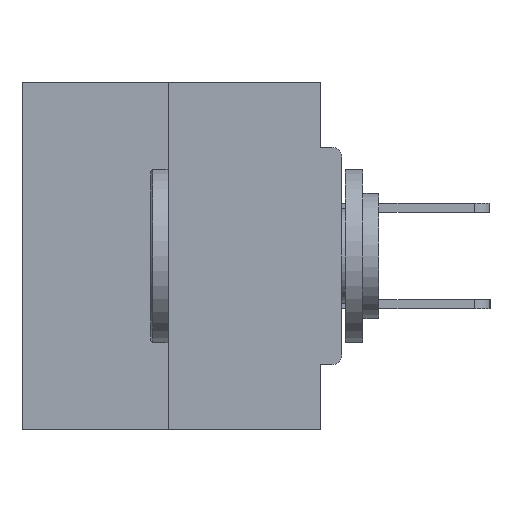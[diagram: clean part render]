
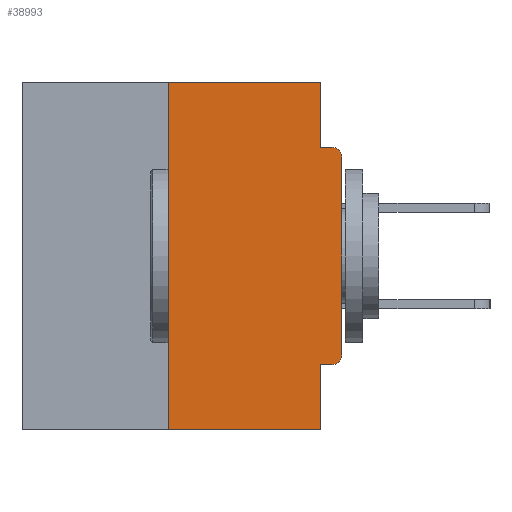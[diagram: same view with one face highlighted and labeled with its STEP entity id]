
A CAD part, left-side view. The second image highlights one B-rep face of the part: STEP entity #38993.
In plain terms, the highlighted planar face has unit normal (-1, 0, 0).
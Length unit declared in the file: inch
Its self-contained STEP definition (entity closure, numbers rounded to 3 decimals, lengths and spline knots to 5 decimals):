
#221 = ORIENTED_EDGE ( 'NONE', *, *, #35527, .T. ) ;
#1279 = ORIENTED_EDGE ( 'NONE', *, *, #10963, .F. ) ;
#2219 = CARTESIAN_POINT ( 'NONE',  ( 0., 0.46, 0. ) ) ;
#2392 = VERTEX_POINT ( 'NONE', #35817 ) ;
#2766 = EDGE_CURVE ( 'NONE', #2392, #14048, #25128, .T. ) ;
#2801 = CIRCLE ( 'NONE', #18973, 0.015 ) ;
#2905 = CARTESIAN_POINT ( 'NONE',  ( 0., 0., 0. ) ) ;
#4479 = ORIENTED_EDGE ( 'NONE', *, *, #8475, .F. ) ;
#4481 = CARTESIAN_POINT ( 'NONE',  ( 0., 0.015, -0.3915 ) ) ;
#5350 = ORIENTED_EDGE ( 'NONE', *, *, #27607, .T. ) ;
#5554 = FACE_OUTER_BOUND ( 'NONE', #33167, .T. ) ;
#7343 = CARTESIAN_POINT ( 'NONE',  ( 0., 0.015, -0.0935 ) ) ;
#8475 = EDGE_CURVE ( 'NONE', #9033, #37160, #33747, .T. ) ;
#9033 = VERTEX_POINT ( 'NONE', #37750 ) ;
#10115 = DIRECTION ( 'NONE',  ( 0., 0., -1. ) ) ;
#10771 = DIRECTION ( 'NONE',  ( 0., 1., 0. ) ) ;
#10941 = DIRECTION ( 'NONE',  ( 0., 0., -1. ) ) ;
#10963 = EDGE_CURVE ( 'NONE', #17591, #20690, #32043, .T. ) ;
#11376 = LINE ( 'NONE', #23255, #17923 ) ;
#11535 = EDGE_CURVE ( 'NONE', #39991, #20321, #31551, .T. ) ;
#11856 = CARTESIAN_POINT ( 'NONE',  ( 0., 0.031, -0.5 ) ) ;
#12567 = ORIENTED_EDGE ( 'NONE', *, *, #33203, .F. ) ;
#12616 = DIRECTION ( 'NONE',  ( 0., 0., -1. ) ) ;
#12732 = DIRECTION ( 'NONE',  ( 0., 0., -1. ) ) ;
#12883 = CARTESIAN_POINT ( 'NONE',  ( 0., 0.031, 0. ) ) ;
#13154 = AXIS2_PLACEMENT_3D ( 'NONE', #2219, #15579, #12732 ) ;
#13315 = DIRECTION ( 'NONE',  ( 0., 0., 1. ) ) ;
#13701 = CARTESIAN_POINT ( 'NONE',  ( 0., 0.015, -0.4065 ) ) ;
#13846 = EDGE_CURVE ( 'NONE', #20321, #39952, #15249, .T. ) ;
#14048 = VERTEX_POINT ( 'NONE', #7343 ) ;
#15249 = LINE ( 'NONE', #2905, #29307 ) ;
#15579 = DIRECTION ( 'NONE',  ( 1., 0., 0. ) ) ;
#15753 = CARTESIAN_POINT ( 'NONE',  ( 0., 0., -0.0935 ) ) ;
#15864 = CARTESIAN_POINT ( 'NONE',  ( 0., 0.25, -0.5 ) ) ;
#15927 = ORIENTED_EDGE ( 'NONE', *, *, #2766, .F. ) ;
#17042 = VECTOR ( 'NONE', #32175, 39.37008 ) ;
#17215 = VECTOR ( 'NONE', #10771, 39.37008 ) ;
#17591 = VERTEX_POINT ( 'NONE', #15864 ) ;
#17923 = VECTOR ( 'NONE', #10115, 39.37008 ) ;
#18106 = PLANE ( 'NONE',  #13154 ) ;
#18656 = CARTESIAN_POINT ( 'NONE',  ( 0., 0.015, -0.1085 ) ) ;
#18973 = AXIS2_PLACEMENT_3D ( 'NONE', #18656, #25163, #12616 ) ;
#19751 = LINE ( 'NONE', #40129, #17215 ) ;
#20080 = ORIENTED_EDGE ( 'NONE', *, *, #13846, .T. ) ;
#20321 = VERTEX_POINT ( 'NONE', #40772 ) ;
#20690 = VERTEX_POINT ( 'NONE', #23132 ) ;
#21570 = CARTESIAN_POINT ( 'NONE',  ( 0., 0.031, -0.5 ) ) ;
#22344 = CARTESIAN_POINT ( 'NONE',  ( 0., 0.25, 0. ) ) ;
#23097 = EDGE_CURVE ( 'NONE', #39991, #9033, #19751, .T. ) ;
#23132 = CARTESIAN_POINT ( 'NONE',  ( 0., 0.25, 0. ) ) ;
#23186 = LINE ( 'NONE', #34841, #28696 ) ;
#23255 = CARTESIAN_POINT ( 'NONE',  ( 0., 0.031, 0. ) ) ;
#25128 = LINE ( 'NONE', #15753, #17042 ) ;
#25163 = DIRECTION ( 'NONE',  ( -1., 0., 0. ) ) ;
#25330 = DIRECTION ( 'NONE',  ( 0., -1., 0. ) ) ;
#26203 = AXIS2_PLACEMENT_3D ( 'NONE', #4481, #30512, #10941 ) ;
#27607 = EDGE_CURVE ( 'NONE', #39952, #14048, #2801, .T. ) ;
#27826 = DIRECTION ( 'NONE',  ( 0., -1., 0. ) ) ;
#27831 = VERTEX_POINT ( 'NONE', #12883 ) ;
#28696 = VECTOR ( 'NONE', #25330, 39.37008 ) ;
#29035 = ORIENTED_EDGE ( 'NONE', *, *, #35840, .F. ) ;
#29307 = VECTOR ( 'NONE', #37598, 39.37008 ) ;
#29528 = VECTOR ( 'NONE', #27826, 39.37008 ) ;
#30512 = DIRECTION ( 'NONE',  ( -1., 0., 0. ) ) ;
#31551 = CIRCLE ( 'NONE', #26203, 0.015 ) ;
#32043 = LINE ( 'NONE', #22344, #33033 ) ;
#32175 = DIRECTION ( 'NONE',  ( 0., -1., 0. ) ) ;
#33033 = VECTOR ( 'NONE', #13315, 39.37008 ) ;
#33089 = CARTESIAN_POINT ( 'NONE',  ( 0., 0., -0.1085 ) ) ;
#33167 = EDGE_LOOP ( 'NONE', ( #12567, #1279, #221, #4479, #39056, #38134, #20080, #5350, #15927, #29035 ) ) ;
#33203 = EDGE_CURVE ( 'NONE', #20690, #27831, #23186, .T. ) ;
#33747 = LINE ( 'NONE', #11856, #39248 ) ;
#33818 = CARTESIAN_POINT ( 'NONE',  ( 0., 0.46, -0.5 ) ) ;
#34841 = CARTESIAN_POINT ( 'NONE',  ( 0., 0.46, 0. ) ) ;
#35314 = DIRECTION ( 'NONE',  ( 0., 0., -1. ) ) ;
#35527 = EDGE_CURVE ( 'NONE', #17591, #37160, #38040, .T. ) ;
#35817 = CARTESIAN_POINT ( 'NONE',  ( 0., 0.031, -0.0935 ) ) ;
#35840 = EDGE_CURVE ( 'NONE', #27831, #2392, #11376, .T. ) ;
#37160 = VERTEX_POINT ( 'NONE', #21570 ) ;
#37598 = DIRECTION ( 'NONE',  ( 0., 0., 1. ) ) ;
#37750 = CARTESIAN_POINT ( 'NONE',  ( 0., 0.031, -0.4065 ) ) ;
#38040 = LINE ( 'NONE', #33818, #29528 ) ;
#38134 = ORIENTED_EDGE ( 'NONE', *, *, #11535, .T. ) ;
#38993 = ADVANCED_FACE ( 'NONE', ( #5554 ), #18106, .F. ) ;
#39056 = ORIENTED_EDGE ( 'NONE', *, *, #23097, .F. ) ;
#39248 = VECTOR ( 'NONE', #35314, 39.37008 ) ;
#39952 = VERTEX_POINT ( 'NONE', #33089 ) ;
#39991 = VERTEX_POINT ( 'NONE', #13701 ) ;
#40129 = CARTESIAN_POINT ( 'NONE',  ( 0., 0., -0.4065 ) ) ;
#40772 = CARTESIAN_POINT ( 'NONE',  ( 0., 0., -0.3915 ) ) ;
